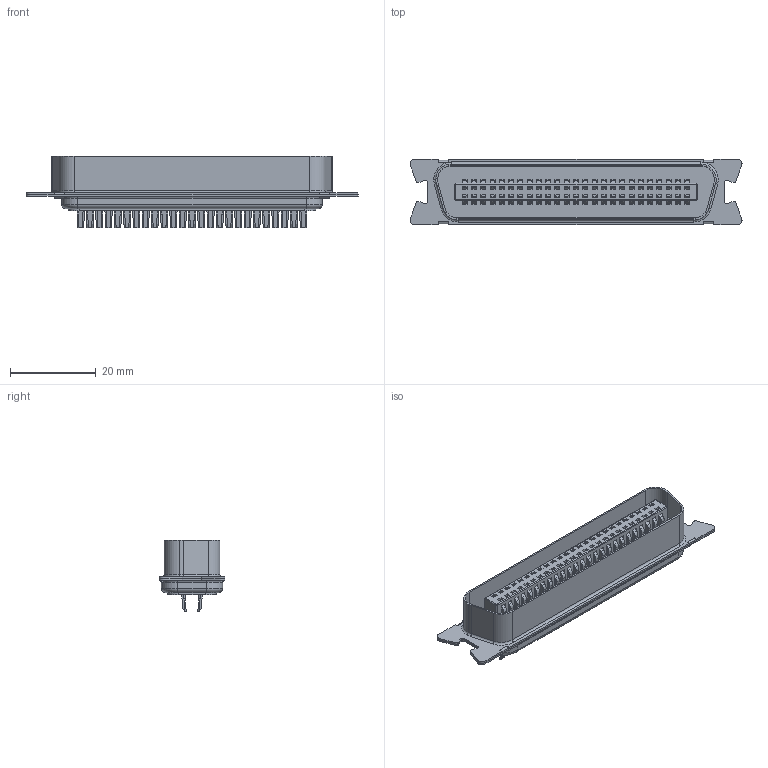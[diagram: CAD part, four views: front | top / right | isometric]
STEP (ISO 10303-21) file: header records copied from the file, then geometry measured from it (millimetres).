
FILE_DESCRIPTION (( 'STEP AP203' ), '1' );
FILE_NAME ('B57-150-622-003.STEP', '2020-06-24T12:39:44', ( '' ), ( '' ), 'SwSTEP 2.0', 'SolidWorks 2020', '' );
FILE_SCHEMA (( 'CONFIG_CONTROL_DESIGN' ));
Products named in the file (5): B57-150-622-003; B57 Contacts MALE_50 Position SOLDER; B57 Front Shell MALE_50 Position LATCH; B57 Back Shell_50 Position LATCH; B57 Housing Insert MALE_50 Position UP
Assembly tree (4 placements, depth 2):
  B57-150-622-003
    B57 Back Shell_50 Position LATCH
    B57 Housing Insert MALE_50 Position UP
    B57 Front Shell MALE_50 Position LATCH
    B57 Contacts MALE_50 Position SOLDER
Bounding box: 77.35 x 15.3 x 16.57 mm (x, y, z)
Volume: 5877.3 mm3; surface area: 14515 mm2
Topology: 53 solids, 53 shells, 5264 faces, 14981 edges, 9524 vertices
Faces by surface type: plane 3806, cylinder 1228, sphere 204, torus 26
Entity records: 168648 total; most frequent: CARTESIAN_POINT 32272, ORIENTED_EDGE 29554, DIRECTION 26809, EDGE_CURVE 14777, LINE 11887, VECTOR 11887, VERTEX_POINT 9524, AXIS2_PLACEMENT_3D 7461
